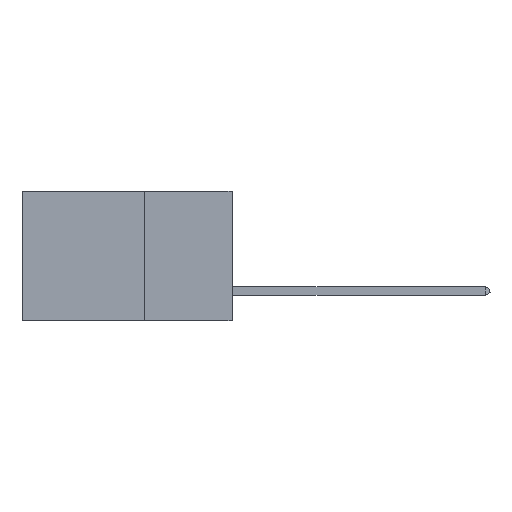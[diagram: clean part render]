
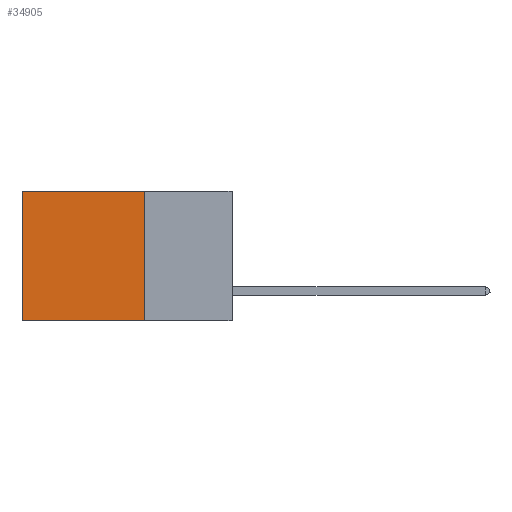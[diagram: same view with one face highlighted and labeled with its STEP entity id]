
A CAD part, left-side view. The second image highlights one B-rep face of the part: STEP entity #34905.
In plain terms, the highlighted planar face has unit normal (-1, 0, 0).
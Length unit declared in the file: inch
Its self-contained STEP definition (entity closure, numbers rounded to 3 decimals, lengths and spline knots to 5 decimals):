
#60 = PLANE ( 'NONE',  #34024 ) ;
#839 = CARTESIAN_POINT ( 'NONE',  ( 0.2875, 0.25, 0. ) ) ;
#2088 = VERTEX_POINT ( 'NONE', #14076 ) ;
#2841 = CARTESIAN_POINT ( 'NONE',  ( 0.2875, 0.6, 0. ) ) ;
#3251 = ORIENTED_EDGE ( 'NONE', *, *, #16152, .F. ) ;
#4796 = ORIENTED_EDGE ( 'NONE', *, *, #45980, .F. ) ;
#6641 = VERTEX_POINT ( 'NONE', #30303 ) ;
#7841 = ORIENTED_EDGE ( 'NONE', *, *, #17070, .T. ) ;
#8483 = CARTESIAN_POINT ( 'NONE',  ( 0.2875, 0.25, 0. ) ) ;
#9135 = DIRECTION ( 'NONE',  ( 0., 1., 0. ) ) ;
#11659 = VECTOR ( 'NONE', #38979, 39.37008 ) ;
#14076 = CARTESIAN_POINT ( 'NONE',  ( 0.2875, 0.25, -0.37 ) ) ;
#14358 = LINE ( 'NONE', #2841, #48213 ) ;
#16152 = EDGE_CURVE ( 'NONE', #2088, #6641, #21159, .T. ) ;
#16705 = VERTEX_POINT ( 'NONE', #33366 ) ;
#17070 = EDGE_CURVE ( 'NONE', #18739, #6641, #14358, .T. ) ;
#18739 = VERTEX_POINT ( 'NONE', #44400 ) ;
#19538 = LINE ( 'NONE', #839, #11659 ) ;
#21159 = LINE ( 'NONE', #44448, #22811 ) ;
#22811 = VECTOR ( 'NONE', #9135, 39.37008 ) ;
#25615 = DIRECTION ( 'NONE',  ( 0., 0., -1. ) ) ;
#26064 = CARTESIAN_POINT ( 'NONE',  ( 0.2875, 0.25, 0. ) ) ;
#27620 = ORIENTED_EDGE ( 'NONE', *, *, #38143, .T. ) ;
#30303 = CARTESIAN_POINT ( 'NONE',  ( 0.2875, 0.6, -0.37 ) ) ;
#31524 = DIRECTION ( 'NONE',  ( 0., 0., -1. ) ) ;
#33366 = CARTESIAN_POINT ( 'NONE',  ( 0.2875, 0.25, 0. ) ) ;
#34024 = AXIS2_PLACEMENT_3D ( 'NONE', #8483, #43303, #31524 ) ;
#34905 = ADVANCED_FACE ( 'NONE', ( #39957 ), #60, .F. ) ;
#37399 = VECTOR ( 'NONE', #49620, 39.37008 ) ;
#38143 = EDGE_CURVE ( 'NONE', #16705, #18739, #38588, .T. ) ;
#38588 = LINE ( 'NONE', #26064, #37399 ) ;
#38979 = DIRECTION ( 'NONE',  ( 0., 0., -1. ) ) ;
#39957 = FACE_OUTER_BOUND ( 'NONE', #40700, .T. ) ;
#40700 = EDGE_LOOP ( 'NONE', ( #7841, #3251, #4796, #27620 ) ) ;
#43303 = DIRECTION ( 'NONE',  ( 1., 0., 0. ) ) ;
#44400 = CARTESIAN_POINT ( 'NONE',  ( 0.2875, 0.6, 0. ) ) ;
#44448 = CARTESIAN_POINT ( 'NONE',  ( 0.2875, 0.25, -0.37 ) ) ;
#45980 = EDGE_CURVE ( 'NONE', #16705, #2088, #19538, .T. ) ;
#48213 = VECTOR ( 'NONE', #25615, 39.37008 ) ;
#49620 = DIRECTION ( 'NONE',  ( 0., 1., 0. ) ) ;
